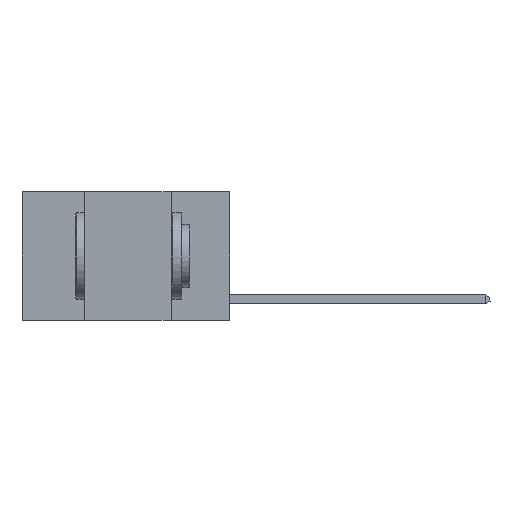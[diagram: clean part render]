
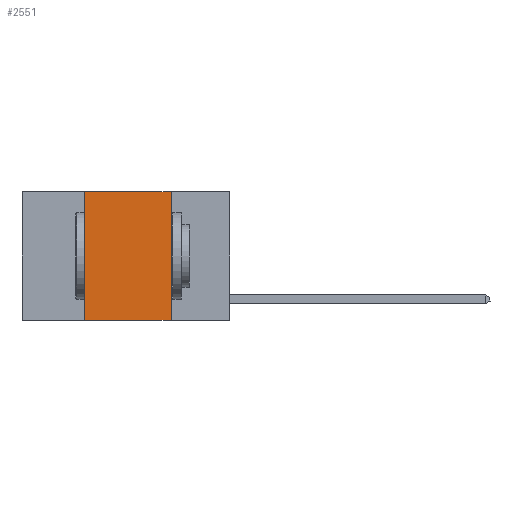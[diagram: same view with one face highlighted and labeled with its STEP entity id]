
A CAD part, left-side view. The second image highlights one B-rep face of the part: STEP entity #2551.
In plain terms, the highlighted planar face has unit normal (-1, 0, 0).
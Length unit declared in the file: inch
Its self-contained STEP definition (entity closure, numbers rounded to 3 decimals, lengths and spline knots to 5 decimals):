
#722 = AXIS2_PLACEMENT_3D ( 'NONE', #15240, #16947, #14460 ) ;
#873 = CARTESIAN_POINT ( 'NONE',  ( 0., 0.17, 0. ) ) ;
#2038 = LINE ( 'NONE', #15725, #14689 ) ;
#2551 = ADVANCED_FACE ( 'NONE', ( #4438 ), #8725, .F. ) ;
#2774 = ORIENTED_EDGE ( 'NONE', *, *, #15509, .F. ) ;
#2887 = CARTESIAN_POINT ( 'NONE',  ( 0., 0.17, -0.37 ) ) ;
#3642 = VECTOR ( 'NONE', #11651, 39.37008 ) ;
#3928 = ORIENTED_EDGE ( 'NONE', *, *, #13736, .T. ) ;
#4438 = FACE_OUTER_BOUND ( 'NONE', #13483, .T. ) ;
#5243 = VERTEX_POINT ( 'NONE', #15029 ) ;
#5771 = VERTEX_POINT ( 'NONE', #14727 ) ;
#6307 = VECTOR ( 'NONE', #15663, 39.37008 ) ;
#6478 = VERTEX_POINT ( 'NONE', #2887 ) ;
#7042 = VECTOR ( 'NONE', #8359, 39.37008 ) ;
#8359 = DIRECTION ( 'NONE',  ( 0., 0., 1. ) ) ;
#8725 = PLANE ( 'NONE',  #722 ) ;
#9448 = EDGE_CURVE ( 'NONE', #5243, #5771, #17030, .T. ) ;
#9857 = LINE ( 'NONE', #14273, #6307 ) ;
#11140 = LINE ( 'NONE', #873, #3642 ) ;
#11651 = DIRECTION ( 'NONE',  ( 0., 0., -1. ) ) ;
#12484 = EDGE_CURVE ( 'NONE', #16006, #6478, #11140, .T. ) ;
#13483 = EDGE_LOOP ( 'NONE', ( #14216, #2774, #14170, #3928 ) ) ;
#13736 = EDGE_CURVE ( 'NONE', #5243, #6478, #2038, .T. ) ;
#14170 = ORIENTED_EDGE ( 'NONE', *, *, #9448, .F. ) ;
#14216 = ORIENTED_EDGE ( 'NONE', *, *, #12484, .F. ) ;
#14273 = CARTESIAN_POINT ( 'NONE',  ( 0., 0.6, 0. ) ) ;
#14460 = DIRECTION ( 'NONE',  ( 0., 0., -1. ) ) ;
#14689 = VECTOR ( 'NONE', #16933, 39.37008 ) ;
#14727 = CARTESIAN_POINT ( 'NONE',  ( 0., 0.42, 0. ) ) ;
#15029 = CARTESIAN_POINT ( 'NONE',  ( 0., 0.42, -0.37 ) ) ;
#15065 = CARTESIAN_POINT ( 'NONE',  ( 0., 0.42, 0. ) ) ;
#15240 = CARTESIAN_POINT ( 'NONE',  ( 0., 0.6, 0. ) ) ;
#15509 = EDGE_CURVE ( 'NONE', #5771, #16006, #9857, .T. ) ;
#15663 = DIRECTION ( 'NONE',  ( 0., -1., 0. ) ) ;
#15725 = CARTESIAN_POINT ( 'NONE',  ( 0., 0.6, -0.37 ) ) ;
#16006 = VERTEX_POINT ( 'NONE', #16612 ) ;
#16612 = CARTESIAN_POINT ( 'NONE',  ( 0., 0.17, 0. ) ) ;
#16933 = DIRECTION ( 'NONE',  ( 0., -1., 0. ) ) ;
#16947 = DIRECTION ( 'NONE',  ( 1., 0., 0. ) ) ;
#17030 = LINE ( 'NONE', #15065, #7042 ) ;
